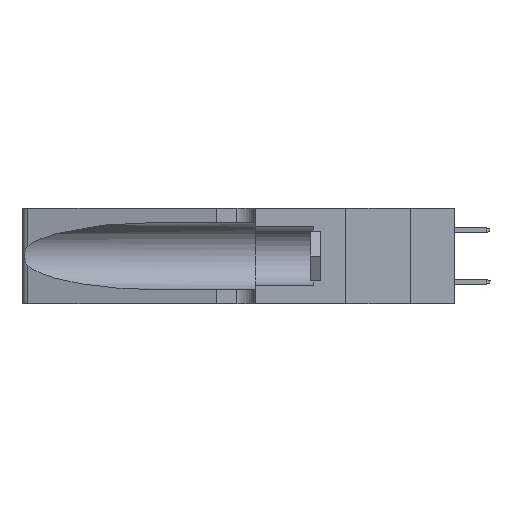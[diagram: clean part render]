
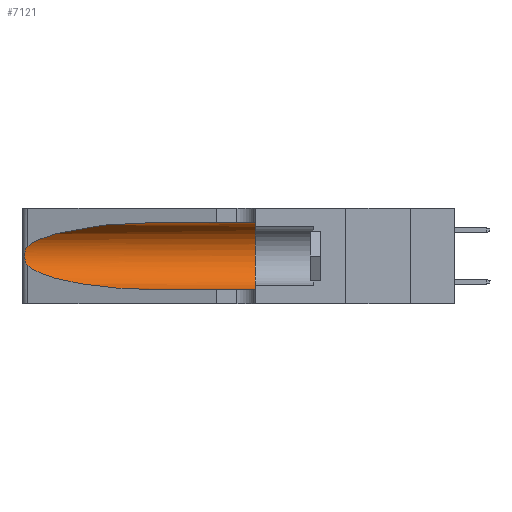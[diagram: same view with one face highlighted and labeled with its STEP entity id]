
A CAD part, left-side view. The second image highlights one B-rep face of the part: STEP entity #7121.
In plain terms, the highlighted cylindrical face has radius 3.308 mm (diameter 6.617 mm), a partial arc.
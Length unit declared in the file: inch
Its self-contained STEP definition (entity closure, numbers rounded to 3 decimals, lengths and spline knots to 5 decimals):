
#72 = CARTESIAN_POINT ( 'NONE',  ( 0.18966, 0.96281, 0.31525 ) ) ;
#104 = CARTESIAN_POINT ( 'NONE',  ( 0.25639, 1.23186, 0.15144 ) ) ;
#376 = VERTEX_POINT ( 'NONE', #8191 ) ;
#461 = ORIENTED_EDGE ( 'NONE', *, *, #11595, .T. ) ;
#2980 = ORIENTED_EDGE ( 'NONE', *, *, #13438, .T. ) ;
#3079 = CARTESIAN_POINT ( 'NONE',  ( 0.26017, 1.23833, 0.17102 ) ) ;
#3603 = EDGE_LOOP ( 'NONE', ( #17739, #15427, #2980, #461, #18959, #13357 ) ) ;
#4252 = CARTESIAN_POINT ( 'NONE',  ( 0.1305, 0.72297, 0.31525 ) ) ;
#4695 = CARTESIAN_POINT ( 'NONE',  ( 0.25487, 1.22718, 0.22369 ) ) ;
#4723 = CARTESIAN_POINT ( 'NONE',  ( 0.26075, 1.23896, 0.19203 ) ) ;
#4737 = CYLINDRICAL_SURFACE ( 'NONE', #15320, 0.13025 ) ;
#5050 = B_SPLINE_CURVE_WITH_KNOTS ( 'NONE', 3,
 ( #11633, #20111, #9666, #16386, #6383, #13086, #4723, #18140, #3079, #9785, #10202, #104, #8664, #11851 ),
 .UNSPECIFIED., .F., .F.,
 ( 4, 2, 2, 2, 2, 2, 4 ),
 ( 0., 0.00027, 0.00053, 0.00107, 0.0016, 0.00187, 0.00214 ),
 .UNSPECIFIED. ) ;
#5206 = VECTOR ( 'NONE', #15914, 39.37008 ) ;
#5402 = LINE ( 'NONE', #13756, #12298 ) ;
#5690 = VERTEX_POINT ( 'NONE', #19489 ) ;
#5918 = CARTESIAN_POINT ( 'NONE',  ( 0.1305, 0.72297, 0.05475 ) ) ;
#6383 = CARTESIAN_POINT ( 'NONE',  ( 0.25854, 1.2359, 0.20912 ) ) ;
#7121 = ADVANCED_FACE ( 'NONE', ( #12874 ), #4737, .F. ) ;
#7535 = CARTESIAN_POINT ( 'NONE',  ( 0.1305, 0.72297, 0.05475 ) ) ;
#7553 = CARTESIAN_POINT ( 'NONE',  ( 0.1305, 0.35, 0.185 ) ) ;
#7702 =( BOUNDED_CURVE ( )  B_SPLINE_CURVE ( 3, ( #4252, #72, #16458, #4695 ),
 .UNSPECIFIED., .F., .F. ) 
 B_SPLINE_CURVE_WITH_KNOTS ( ( 4, 4 ),
 ( 1.5708, 2.84003 ),
 .UNSPECIFIED. ) 
 CURVE ( )  GEOMETRIC_REPRESENTATION_ITEM ( )  RATIONAL_B_SPLINE_CURVE ( ( 1., 0.87, 0.87, 1. ) ) 
 REPRESENTATION_ITEM ( '' )  );
#7837 =( BOUNDED_CURVE ( )  B_SPLINE_CURVE ( 3, ( #20874, #20976, #19221, #5918 ),
 .UNSPECIFIED., .F., .T. ) 
 B_SPLINE_CURVE_WITH_KNOTS ( ( 4, 4 ),
 ( 3.44316, 4.71239 ),
 .UNSPECIFIED. ) 
 CURVE ( )  GEOMETRIC_REPRESENTATION_ITEM ( )  RATIONAL_B_SPLINE_CURVE ( ( 1., 0.87, 0.87, 1. ) ) 
 REPRESENTATION_ITEM ( '' )  );
#7859 = VERTEX_POINT ( 'NONE', #9278 ) ;
#8191 = CARTESIAN_POINT ( 'NONE',  ( 0.25487, 1.22718, 0.14631 ) ) ;
#8664 = CARTESIAN_POINT ( 'NONE',  ( 0.25555, 1.22993, 0.14849 ) ) ;
#9278 = CARTESIAN_POINT ( 'NONE',  ( 0.1305, 0.35, 0.31525 ) ) ;
#9666 = CARTESIAN_POINT ( 'NONE',  ( 0.25639, 1.23184, 0.21858 ) ) ;
#9785 = CARTESIAN_POINT ( 'NONE',  ( 0.25856, 1.23593, 0.16098 ) ) ;
#10202 = CARTESIAN_POINT ( 'NONE',  ( 0.25789, 1.23486, 0.15765 ) ) ;
#10356 = DIRECTION ( 'NONE',  ( 0., -1., 0. ) ) ;
#10744 = CARTESIAN_POINT ( 'NONE',  ( 0.1305, 1.61858, 0.31525 ) ) ;
#10879 = CARTESIAN_POINT ( 'NONE',  ( 0.1305, 0.72297, 0.31525 ) ) ;
#11446 = DIRECTION ( 'NONE',  ( 0., -1., 0. ) ) ;
#11595 = EDGE_CURVE ( 'NONE', #12628, #18989, #5402, .T. ) ;
#11633 = CARTESIAN_POINT ( 'NONE',  ( 0.25487, 1.22718, 0.22369 ) ) ;
#11851 = CARTESIAN_POINT ( 'NONE',  ( 0.25487, 1.22718, 0.14631 ) ) ;
#12298 = VECTOR ( 'NONE', #10356, 39.37008 ) ;
#12628 = VERTEX_POINT ( 'NONE', #7535 ) ;
#12874 = FACE_OUTER_BOUND ( 'NONE', #3603, .T. ) ;
#13086 = CARTESIAN_POINT ( 'NONE',  ( 0.26018, 1.23835, 0.19895 ) ) ;
#13357 = ORIENTED_EDGE ( 'NONE', *, *, #19576, .F. ) ;
#13438 = EDGE_CURVE ( 'NONE', #376, #12628, #7837, .T. ) ;
#13756 = CARTESIAN_POINT ( 'NONE',  ( 0.1305, 1.61858, 0.05475 ) ) ;
#14265 = DIRECTION ( 'NONE',  ( 0., 1., 0. ) ) ;
#14373 = LINE ( 'NONE', #10744, #5206 ) ;
#14862 = CARTESIAN_POINT ( 'NONE',  ( 0.1305, 1.61858, 0.185 ) ) ;
#15061 = AXIS2_PLACEMENT_3D ( 'NONE', #7553, #14265, #20966 ) ;
#15320 = AXIS2_PLACEMENT_3D ( 'NONE', #14862, #11446, #19918 ) ;
#15427 = ORIENTED_EDGE ( 'NONE', *, *, #19388, .T. ) ;
#15914 = DIRECTION ( 'NONE',  ( 0., -1., 0. ) ) ;
#16386 = CARTESIAN_POINT ( 'NONE',  ( 0.25787, 1.23484, 0.2124 ) ) ;
#16458 = CARTESIAN_POINT ( 'NONE',  ( 0.2373, 1.15595, 0.28018 ) ) ;
#16928 = CARTESIAN_POINT ( 'NONE',  ( 0.1305, 0.35, 0.05475 ) ) ;
#17081 = EDGE_CURVE ( 'NONE', #19187, #5690, #7702, .T. ) ;
#17739 = ORIENTED_EDGE ( 'NONE', *, *, #17081, .T. ) ;
#18140 = CARTESIAN_POINT ( 'NONE',  ( 0.26075, 1.23896, 0.178 ) ) ;
#18198 = EDGE_CURVE ( 'NONE', #7859, #18989, #20315, .T. ) ;
#18959 = ORIENTED_EDGE ( 'NONE', *, *, #18198, .F. ) ;
#18989 = VERTEX_POINT ( 'NONE', #16928 ) ;
#19187 = VERTEX_POINT ( 'NONE', #10879 ) ;
#19221 = CARTESIAN_POINT ( 'NONE',  ( 0.18966, 0.96281, 0.05475 ) ) ;
#19388 = EDGE_CURVE ( 'NONE', #5690, #376, #5050, .T. ) ;
#19489 = CARTESIAN_POINT ( 'NONE',  ( 0.25487, 1.22718, 0.22369 ) ) ;
#19576 = EDGE_CURVE ( 'NONE', #19187, #7859, #14373, .T. ) ;
#19918 = DIRECTION ( 'NONE',  ( 0., 0., -1. ) ) ;
#20111 = CARTESIAN_POINT ( 'NONE',  ( 0.25555, 1.22994, 0.2215 ) ) ;
#20315 = CIRCLE ( 'NONE', #15061, 0.13025 ) ;
#20874 = CARTESIAN_POINT ( 'NONE',  ( 0.25487, 1.22718, 0.14631 ) ) ;
#20966 = DIRECTION ( 'NONE',  ( 0., 0., 1. ) ) ;
#20976 = CARTESIAN_POINT ( 'NONE',  ( 0.2373, 1.15595, 0.08982 ) ) ;
